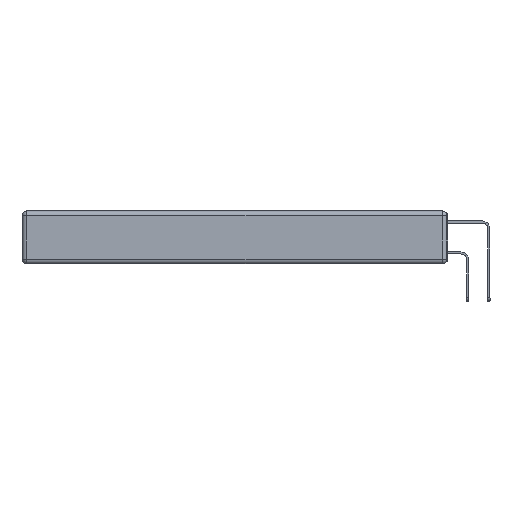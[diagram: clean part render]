
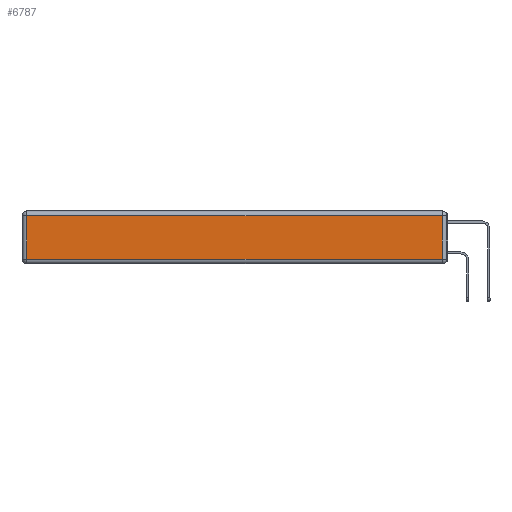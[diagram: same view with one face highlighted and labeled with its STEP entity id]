
A CAD part, left-side view. The second image highlights one B-rep face of the part: STEP entity #6787.
In plain terms, the highlighted planar face has unit normal (-1, 0, 0).
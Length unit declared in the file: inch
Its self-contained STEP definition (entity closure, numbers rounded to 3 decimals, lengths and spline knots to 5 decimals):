
#448 = EDGE_CURVE ( 'NONE', #2893, #22173, #16209, .T. ) ;
#844 = CARTESIAN_POINT ( 'NONE',  ( 0., 0., -0.313 ) ) ;
#913 = CARTESIAN_POINT ( 'NONE',  ( 0., 0., -0.343 ) ) ;
#1162 = DIRECTION ( 'NONE',  ( 0., 0., -1. ) ) ;
#1245 = VECTOR ( 'NONE', #3824, 39.37008 ) ;
#1594 = LINE ( 'NONE', #24365, #1245 ) ;
#2893 = VERTEX_POINT ( 'NONE', #6950 ) ;
#3611 = ORIENTED_EDGE ( 'NONE', *, *, #6092, .T. ) ;
#3824 = DIRECTION ( 'NONE',  ( 0., 1., 0. ) ) ;
#4470 = VERTEX_POINT ( 'NONE', #21924 ) ;
#4786 = DIRECTION ( 'NONE',  ( -1., 0., 0. ) ) ;
#4985 = VECTOR ( 'NONE', #12661, 39.37008 ) ;
#5033 = PLANE ( 'NONE',  #22485 ) ;
#5816 = ORIENTED_EDGE ( 'NONE', *, *, #23414, .T. ) ;
#6092 = EDGE_CURVE ( 'NONE', #12026, #4470, #1594, .T. ) ;
#6787 = ADVANCED_FACE ( 'NONE', ( #21915 ), #5033, .T. ) ;
#6950 = CARTESIAN_POINT ( 'NONE',  ( 0., 2.72, -0.313 ) ) ;
#8550 = CARTESIAN_POINT ( 'NONE',  ( 0., 0.03, -0.343 ) ) ;
#12026 = VERTEX_POINT ( 'NONE', #18196 ) ;
#12205 = VECTOR ( 'NONE', #23732, 39.37008 ) ;
#12661 = DIRECTION ( 'NONE',  ( 0., 0., 1. ) ) ;
#12930 = EDGE_LOOP ( 'NONE', ( #22707, #19647, #3611, #5816 ) ) ;
#13761 = EDGE_CURVE ( 'NONE', #22173, #12026, #19806, .T. ) ;
#15022 = VECTOR ( 'NONE', #1162, 39.37008 ) ;
#16209 = LINE ( 'NONE', #844, #12205 ) ;
#16405 = CARTESIAN_POINT ( 'NONE',  ( 0., 2.72, -0.343 ) ) ;
#18196 = CARTESIAN_POINT ( 'NONE',  ( 0., 0.03, -0.03 ) ) ;
#18420 = LINE ( 'NONE', #16405, #15022 ) ;
#19647 = ORIENTED_EDGE ( 'NONE', *, *, #13761, .T. ) ;
#19806 = LINE ( 'NONE', #8550, #4985 ) ;
#20297 = DIRECTION ( 'NONE',  ( 0., 0., 1. ) ) ;
#21915 = FACE_OUTER_BOUND ( 'NONE', #12930, .T. ) ;
#21924 = CARTESIAN_POINT ( 'NONE',  ( 0., 2.72, -0.03 ) ) ;
#22173 = VERTEX_POINT ( 'NONE', #23242 ) ;
#22485 = AXIS2_PLACEMENT_3D ( 'NONE', #913, #4786, #20297 ) ;
#22707 = ORIENTED_EDGE ( 'NONE', *, *, #448, .T. ) ;
#23242 = CARTESIAN_POINT ( 'NONE',  ( 0., 0.03, -0.313 ) ) ;
#23414 = EDGE_CURVE ( 'NONE', #4470, #2893, #18420, .T. ) ;
#23732 = DIRECTION ( 'NONE',  ( 0., -1., 0. ) ) ;
#24365 = CARTESIAN_POINT ( 'NONE',  ( 0., 2.75, -0.03 ) ) ;
